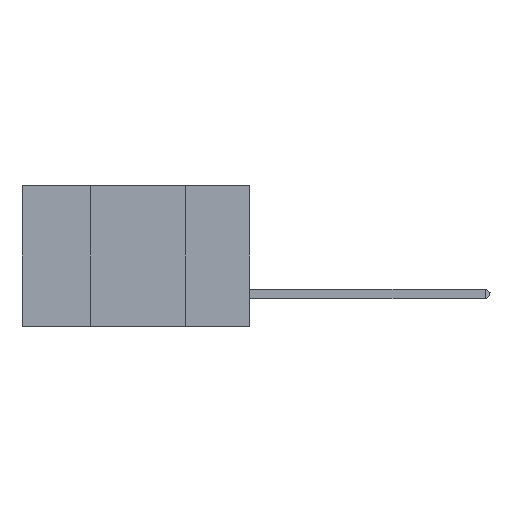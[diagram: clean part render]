
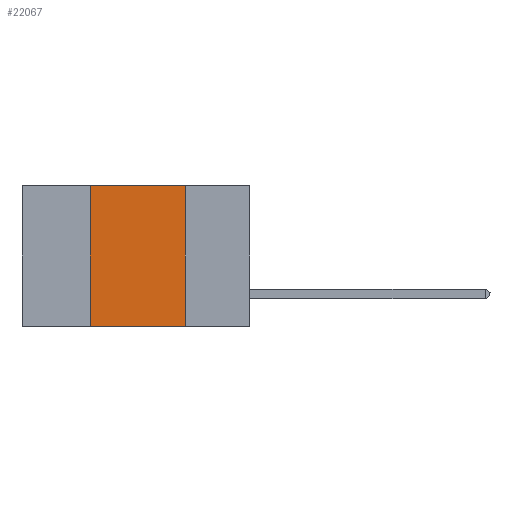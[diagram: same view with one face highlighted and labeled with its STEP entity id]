
A CAD part, left-side view. The second image highlights one B-rep face of the part: STEP entity #22067.
In plain terms, the highlighted planar face has unit normal (-1, 0, 0).
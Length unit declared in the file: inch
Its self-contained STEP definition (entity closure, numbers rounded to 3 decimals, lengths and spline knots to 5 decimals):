
#1325 = CARTESIAN_POINT ( 'NONE',  ( 0., 0.17, -0.37 ) ) ;
#1448 = LINE ( 'NONE', #16868, #11968 ) ;
#2525 = VECTOR ( 'NONE', #10449, 39.37008 ) ;
#3055 = LINE ( 'NONE', #21600, #6352 ) ;
#4141 = VECTOR ( 'NONE', #10648, 39.37008 ) ;
#4460 = ORIENTED_EDGE ( 'NONE', *, *, #15950, .F. ) ;
#5380 = DIRECTION ( 'NONE',  ( 0., 0., 1. ) ) ;
#5465 = CARTESIAN_POINT ( 'NONE',  ( 0., 0.17, 0. ) ) ;
#6076 = CARTESIAN_POINT ( 'NONE',  ( 0., 0.17, 0. ) ) ;
#6352 = VECTOR ( 'NONE', #11992, 39.37008 ) ;
#6923 = VERTEX_POINT ( 'NONE', #22196 ) ;
#8242 = CARTESIAN_POINT ( 'NONE',  ( 0., 0.6, 0. ) ) ;
#8541 = EDGE_CURVE ( 'NONE', #18588, #14449, #12767, .T. ) ;
#9078 = FACE_OUTER_BOUND ( 'NONE', #22544, .T. ) ;
#9292 = VERTEX_POINT ( 'NONE', #16340 ) ;
#9548 = LINE ( 'NONE', #23231, #4141 ) ;
#9855 = DIRECTION ( 'NONE',  ( 0., 0., -1. ) ) ;
#10033 = ORIENTED_EDGE ( 'NONE', *, *, #10200, .T. ) ;
#10200 = EDGE_CURVE ( 'NONE', #6923, #14449, #3055, .T. ) ;
#10300 = ORIENTED_EDGE ( 'NONE', *, *, #8541, .F. ) ;
#10449 = DIRECTION ( 'NONE',  ( 0., 0., -1. ) ) ;
#10648 = DIRECTION ( 'NONE',  ( 0., -1., 0. ) ) ;
#11968 = VECTOR ( 'NONE', #5380, 39.37008 ) ;
#11992 = DIRECTION ( 'NONE',  ( 0., -1., 0. ) ) ;
#12028 = PLANE ( 'NONE',  #21775 ) ;
#12767 = LINE ( 'NONE', #6076, #2525 ) ;
#14449 = VERTEX_POINT ( 'NONE', #1325 ) ;
#15950 = EDGE_CURVE ( 'NONE', #6923, #9292, #1448, .T. ) ;
#16222 = EDGE_CURVE ( 'NONE', #9292, #18588, #9548, .T. ) ;
#16340 = CARTESIAN_POINT ( 'NONE',  ( 0., 0.42, 0. ) ) ;
#16868 = CARTESIAN_POINT ( 'NONE',  ( 0., 0.42, 0. ) ) ;
#18210 = ORIENTED_EDGE ( 'NONE', *, *, #16222, .F. ) ;
#18588 = VERTEX_POINT ( 'NONE', #5465 ) ;
#21600 = CARTESIAN_POINT ( 'NONE',  ( 0., 0.6, -0.37 ) ) ;
#21716 = DIRECTION ( 'NONE',  ( 1., 0., 0. ) ) ;
#21775 = AXIS2_PLACEMENT_3D ( 'NONE', #8242, #21716, #9855 ) ;
#22067 = ADVANCED_FACE ( 'NONE', ( #9078 ), #12028, .F. ) ;
#22196 = CARTESIAN_POINT ( 'NONE',  ( 0., 0.42, -0.37 ) ) ;
#22544 = EDGE_LOOP ( 'NONE', ( #10300, #18210, #4460, #10033 ) ) ;
#23231 = CARTESIAN_POINT ( 'NONE',  ( 0., 0.6, 0. ) ) ;
